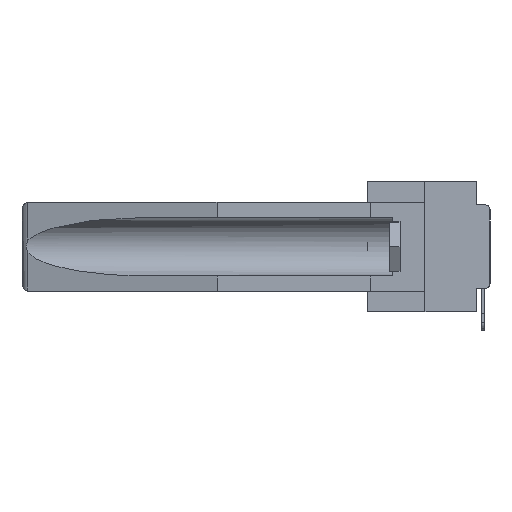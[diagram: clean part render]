
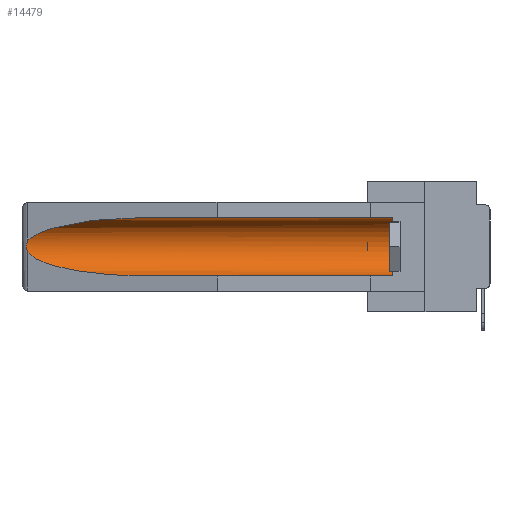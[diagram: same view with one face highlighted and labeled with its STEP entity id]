
A CAD part, left-side view. The second image highlights one B-rep face of the part: STEP entity #14479.
In plain terms, the highlighted cylindrical face has radius 2.857 mm (diameter 5.715 mm), a partial arc.
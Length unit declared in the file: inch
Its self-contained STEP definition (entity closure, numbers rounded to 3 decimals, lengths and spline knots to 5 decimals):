
#2398 = CIRCLE ( 'NONE', #31902, 0.1125 ) ;
#2556 = EDGE_CURVE ( 'NONE', #9984, #39721, #4591, .T. ) ;
#3173 = CARTESIAN_POINT ( 'NONE',  ( 0.26597, 1.5296, -0.19026 ) ) ;
#4480 = CARTESIAN_POINT ( 'NONE',  ( 0.155, 0.126, -0.059 ) ) ;
#4591 =( BOUNDED_CURVE ( )  B_SPLINE_CURVE ( 3, ( #24527, #40068, #36924, #11530 ),
 .UNSPECIFIED., .F., .F. ) 
 B_SPLINE_CURVE_WITH_KNOTS ( ( 4, 4 ),
 ( 0.1948, 1.5708 ),
 .UNSPECIFIED. ) 
 CURVE ( )  GEOMETRIC_REPRESENTATION_ITEM ( )  RATIONAL_B_SPLINE_CURVE ( ( 1., 0.848, 0.848, 1. ) ) 
 REPRESENTATION_ITEM ( '' )  );
#6228 = CARTESIAN_POINT ( 'NONE',  ( 0.26655, 1.53094, -0.18657 ) ) ;
#6305 = CYLINDRICAL_SURFACE ( 'NONE', #36656, 0.1125 ) ;
#6338 = CARTESIAN_POINT ( 'NONE',  ( 0.155, 1.07973, -0.059 ) ) ;
#6654 = VECTOR ( 'NONE', #20951, 39.37008 ) ;
#7843 = ORIENTED_EDGE ( 'NONE', *, *, #23554, .F. ) ;
#8761 = CARTESIAN_POINT ( 'NONE',  ( 0.21114, 1.30732, -0.059 ) ) ;
#9366 = CARTESIAN_POINT ( 'NONE',  ( 0.26654, 1.53092, -0.15636 ) ) ;
#9784 = CARTESIAN_POINT ( 'NONE',  ( 0.26537, 1.52718, -0.14972 ) ) ;
#9984 = VERTEX_POINT ( 'NONE', #28169 ) ;
#10198 = DIRECTION ( 'NONE',  ( 0., 1., 0. ) ) ;
#10583 = EDGE_CURVE ( 'NONE', #16427, #22844, #12700, .T. ) ;
#11530 = CARTESIAN_POINT ( 'NONE',  ( 0.155, 1.07973, -0.284 ) ) ;
#12700 =( BOUNDED_CURVE ( )  B_SPLINE_CURVE ( 3, ( #6338, #8761, #15971, #15581 ),
 .UNSPECIFIED., .F., .F. ) 
 B_SPLINE_CURVE_WITH_KNOTS ( ( 4, 4 ),
 ( 4.71239, 6.08839 ),
 .UNSPECIFIED. ) 
 CURVE ( )  GEOMETRIC_REPRESENTATION_ITEM ( )  RATIONAL_B_SPLINE_CURVE ( ( 1., 0.848, 0.848, 1. ) ) 
 REPRESENTATION_ITEM ( '' )  );
#14479 = ADVANCED_FACE ( 'NONE', ( #34456 ), #6305, .F. ) ;
#15163 = VECTOR ( 'NONE', #36969, 39.37008 ) ;
#15330 = CARTESIAN_POINT ( 'NONE',  ( 0.2675, 1.53308, -0.17534 ) ) ;
#15581 = CARTESIAN_POINT ( 'NONE',  ( 0.26537, 1.52718, -0.14972 ) ) ;
#15859 = CARTESIAN_POINT ( 'NONE',  ( 0.2673, 1.53269, -0.17917 ) ) ;
#15971 = CARTESIAN_POINT ( 'NONE',  ( 0.25451, 1.48313, -0.09465 ) ) ;
#16427 = VERTEX_POINT ( 'NONE', #38882 ) ;
#16722 = CARTESIAN_POINT ( 'NONE',  ( 0.155, 0.126, -0.1715 ) ) ;
#17017 = ORIENTED_EDGE ( 'NONE', *, *, #38681, .T. ) ;
#17302 = EDGE_CURVE ( 'NONE', #22844, #9984, #30908, .T. ) ;
#18164 = VERTEX_POINT ( 'NONE', #4480 ) ;
#18341 = CARTESIAN_POINT ( 'NONE',  ( 0.155, 1.07973, -0.284 ) ) ;
#19867 = ORIENTED_EDGE ( 'NONE', *, *, #17302, .T. ) ;
#20951 = DIRECTION ( 'NONE',  ( 0., 1., 0. ) ) ;
#21564 = LINE ( 'NONE', #30605, #15163 ) ;
#21930 = CARTESIAN_POINT ( 'NONE',  ( 0.2673, 1.5327, -0.16383 ) ) ;
#22070 = CARTESIAN_POINT ( 'NONE',  ( 0.26537, 1.52718, -0.14972 ) ) ;
#22844 = VERTEX_POINT ( 'NONE', #9784 ) ;
#23044 = VERTEX_POINT ( 'NONE', #31219 ) ;
#23437 = LINE ( 'NONE', #37232, #6654 ) ;
#23554 = EDGE_CURVE ( 'NONE', #23044, #39721, #23437, .T. ) ;
#24527 = CARTESIAN_POINT ( 'NONE',  ( 0.26537, 1.52718, -0.19328 ) ) ;
#25696 = CARTESIAN_POINT ( 'NONE',  ( 0.155, -0.30754, -0.1715 ) ) ;
#26679 = DIRECTION ( 'NONE',  ( 0., -1., 0. ) ) ;
#28169 = CARTESIAN_POINT ( 'NONE',  ( 0.26537, 1.52718, -0.19328 ) ) ;
#30605 = CARTESIAN_POINT ( 'NONE',  ( 0.155, -0.30754, -0.059 ) ) ;
#30908 = B_SPLINE_CURVE_WITH_KNOTS ( 'NONE', 3,
 ( #22070, #31605, #9366, #21930, #34773, #15330, #15859, #6228, #3173, #40690 ),
 .UNSPECIFIED., .F., .F.,
 ( 4, 2, 2, 2, 4 ),
 ( 0., 0.00029, 0.00058, 0.00087, 0.00117 ),
 .UNSPECIFIED. ) ;
#31072 = ORIENTED_EDGE ( 'NONE', *, *, #2556, .T. ) ;
#31219 = CARTESIAN_POINT ( 'NONE',  ( 0.155, 0.126, -0.284 ) ) ;
#31507 = EDGE_LOOP ( 'NONE', ( #38706, #19867, #31072, #7843, #17017, #35721 ) ) ;
#31605 = CARTESIAN_POINT ( 'NONE',  ( 0.26597, 1.52961, -0.15275 ) ) ;
#31902 = AXIS2_PLACEMENT_3D ( 'NONE', #16722, #26679, #38775 ) ;
#32276 = DIRECTION ( 'NONE',  ( 0., 0., 1. ) ) ;
#34456 = FACE_OUTER_BOUND ( 'NONE', #31507, .T. ) ;
#34773 = CARTESIAN_POINT ( 'NONE',  ( 0.2675, 1.53308, -0.16763 ) ) ;
#35721 = ORIENTED_EDGE ( 'NONE', *, *, #39723, .T. ) ;
#36656 = AXIS2_PLACEMENT_3D ( 'NONE', #25696, #10198, #32276 ) ;
#36924 = CARTESIAN_POINT ( 'NONE',  ( 0.21114, 1.30732, -0.284 ) ) ;
#36969 = DIRECTION ( 'NONE',  ( 0., 1., 0. ) ) ;
#37232 = CARTESIAN_POINT ( 'NONE',  ( 0.155, -0.30754, -0.284 ) ) ;
#38681 = EDGE_CURVE ( 'NONE', #23044, #18164, #2398, .T. ) ;
#38706 = ORIENTED_EDGE ( 'NONE', *, *, #10583, .T. ) ;
#38775 = DIRECTION ( 'NONE',  ( 0., 0., 1. ) ) ;
#38882 = CARTESIAN_POINT ( 'NONE',  ( 0.155, 1.07973, -0.059 ) ) ;
#39721 = VERTEX_POINT ( 'NONE', #18341 ) ;
#39723 = EDGE_CURVE ( 'NONE', #18164, #16427, #21564, .T. ) ;
#40068 = CARTESIAN_POINT ( 'NONE',  ( 0.25451, 1.48313, -0.24835 ) ) ;
#40690 = CARTESIAN_POINT ( 'NONE',  ( 0.26537, 1.52718, -0.19328 ) ) ;
